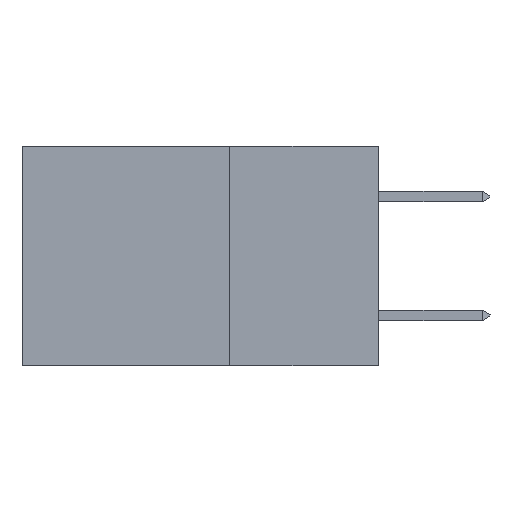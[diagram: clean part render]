
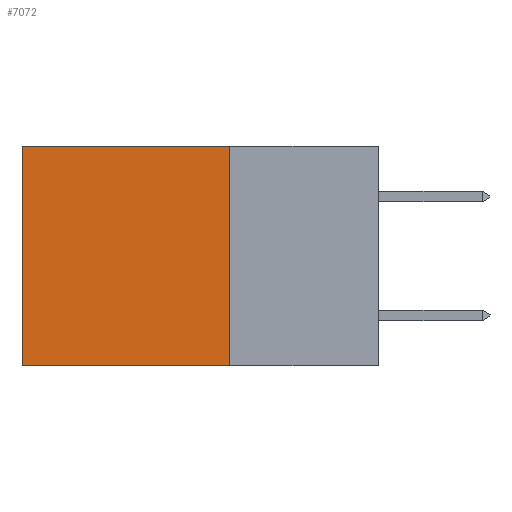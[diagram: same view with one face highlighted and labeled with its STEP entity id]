
A CAD part, left-side view. The second image highlights one B-rep face of the part: STEP entity #7072.
In plain terms, the highlighted planar face has unit normal (-1, 0, 0).
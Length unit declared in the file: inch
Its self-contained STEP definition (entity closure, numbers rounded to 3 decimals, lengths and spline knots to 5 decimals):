
#135 = DIRECTION ( 'NONE',  ( 0., 0., -1. ) ) ;
#312 = CARTESIAN_POINT ( 'NONE',  ( 0.298, 0.25, 0. ) ) ;
#533 = LINE ( 'NONE', #312, #6345 ) ;
#589 = VECTOR ( 'NONE', #135, 39.37008 ) ;
#1069 = DIRECTION ( 'NONE',  ( 0., 0., -1. ) ) ;
#1380 = VECTOR ( 'NONE', #4588, 39.37008 ) ;
#1500 = ORIENTED_EDGE ( 'NONE', *, *, #8269, .F. ) ;
#1576 = LINE ( 'NONE', #9271, #7937 ) ;
#1726 = VERTEX_POINT ( 'NONE', #6739 ) ;
#1987 = CARTESIAN_POINT ( 'NONE',  ( 0.298, 0.25, -0.37 ) ) ;
#2033 = PLANE ( 'NONE',  #8951 ) ;
#2208 = EDGE_CURVE ( 'NONE', #9680, #4469, #8491, .T. ) ;
#2658 = CARTESIAN_POINT ( 'NONE',  ( 0.298, 0.25, -0.37 ) ) ;
#2998 = EDGE_LOOP ( 'NONE', ( #9421, #3529, #1500, #5692 ) ) ;
#3529 = ORIENTED_EDGE ( 'NONE', *, *, #2208, .F. ) ;
#3537 = LINE ( 'NONE', #4990, #589 ) ;
#3580 = DIRECTION ( 'NONE',  ( 0., 1., 0. ) ) ;
#3712 = CARTESIAN_POINT ( 'NONE',  ( 0.298, 0.6, 0. ) ) ;
#4120 = EDGE_CURVE ( 'NONE', #7704, #4469, #1576, .T. ) ;
#4469 = VERTEX_POINT ( 'NONE', #9456 ) ;
#4588 = DIRECTION ( 'NONE',  ( 0., 1., 0. ) ) ;
#4990 = CARTESIAN_POINT ( 'NONE',  ( 0.298, 0.25, 0. ) ) ;
#5692 = ORIENTED_EDGE ( 'NONE', *, *, #5814, .T. ) ;
#5814 = EDGE_CURVE ( 'NONE', #1726, #7704, #533, .T. ) ;
#6024 = DIRECTION ( 'NONE',  ( 1., 0., 0. ) ) ;
#6345 = VECTOR ( 'NONE', #3580, 39.37008 ) ;
#6739 = CARTESIAN_POINT ( 'NONE',  ( 0.298, 0.25, 0. ) ) ;
#7072 = ADVANCED_FACE ( 'NONE', ( #7484 ), #2033, .F. ) ;
#7484 = FACE_OUTER_BOUND ( 'NONE', #2998, .T. ) ;
#7704 = VERTEX_POINT ( 'NONE', #3712 ) ;
#7846 = CARTESIAN_POINT ( 'NONE',  ( 0.298, 0.25, 0. ) ) ;
#7937 = VECTOR ( 'NONE', #10179, 39.37008 ) ;
#8269 = EDGE_CURVE ( 'NONE', #1726, #9680, #3537, .T. ) ;
#8491 = LINE ( 'NONE', #1987, #1380 ) ;
#8951 = AXIS2_PLACEMENT_3D ( 'NONE', #7846, #6024, #1069 ) ;
#9271 = CARTESIAN_POINT ( 'NONE',  ( 0.298, 0.6, 0. ) ) ;
#9421 = ORIENTED_EDGE ( 'NONE', *, *, #4120, .T. ) ;
#9456 = CARTESIAN_POINT ( 'NONE',  ( 0.298, 0.6, -0.37 ) ) ;
#9680 = VERTEX_POINT ( 'NONE', #2658 ) ;
#10179 = DIRECTION ( 'NONE',  ( 0., 0., -1. ) ) ;
